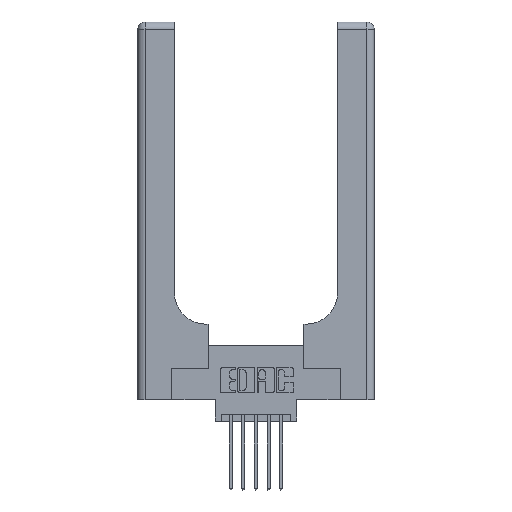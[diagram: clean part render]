
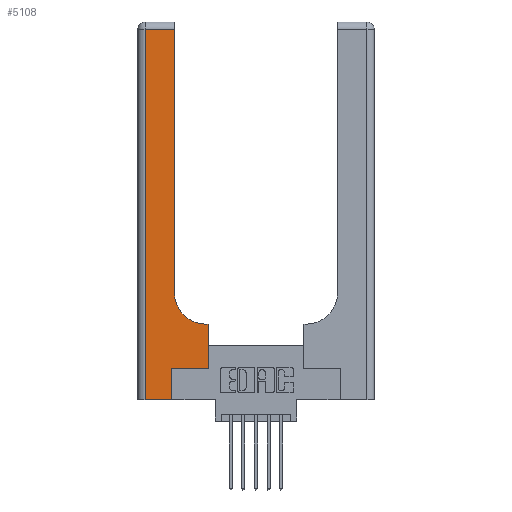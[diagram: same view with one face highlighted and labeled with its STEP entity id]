
A CAD part, top view. The second image highlights one B-rep face of the part: STEP entity #5108.
In plain terms, the highlighted planar face has unit normal (0, 0, 1).
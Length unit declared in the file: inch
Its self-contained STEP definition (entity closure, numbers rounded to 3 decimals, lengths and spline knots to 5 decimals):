
#667 = EDGE_CURVE ( 'NONE', #873, #13312, #13316, .T. ) ;
#873 = VERTEX_POINT ( 'NONE', #10193 ) ;
#890 = VECTOR ( 'NONE', #1889, 39.37008 ) ;
#1004 = VECTOR ( 'NONE', #8299, 39.37008 ) ;
#1135 = DIRECTION ( 'NONE',  ( -1., 0., 0. ) ) ;
#1492 = VECTOR ( 'NONE', #5512, 39.37008 ) ;
#1509 = ORIENTED_EDGE ( 'NONE', *, *, #4184, .T. ) ;
#1645 = CARTESIAN_POINT ( 'NONE',  ( 0.5585, 0.25, 0.37 ) ) ;
#1889 = DIRECTION ( 'NONE',  ( 0., 1., 0. ) ) ;
#2046 = LINE ( 'NONE', #1645, #9063 ) ;
#2167 = EDGE_CURVE ( 'NONE', #13312, #11450, #8857, .T. ) ;
#2388 = CARTESIAN_POINT ( 'NONE',  ( 0.269, 0., 0.37 ) ) ;
#2392 = LINE ( 'NONE', #10535, #1004 ) ;
#2447 = AXIS2_PLACEMENT_3D ( 'NONE', #11686, #13950, #7360 ) ;
#2586 = VERTEX_POINT ( 'NONE', #9330 ) ;
#2750 = DIRECTION ( 'NONE',  ( 0., 1., 0. ) ) ;
#2812 = EDGE_CURVE ( 'NONE', #9667, #2876, #4228, .T. ) ;
#2876 = VERTEX_POINT ( 'NONE', #13076 ) ;
#3674 = CARTESIAN_POINT ( 'NONE',  ( 0.5415, 0.6, 0.37 ) ) ;
#3947 = CARTESIAN_POINT ( 'NONE',  ( 0.2915, 3., 0.37 ) ) ;
#3962 = PLANE ( 'NONE',  #2447 ) ;
#3976 = LINE ( 'NONE', #3947, #890 ) ;
#4128 = CARTESIAN_POINT ( 'NONE',  ( 0.269, 0., 0.37 ) ) ;
#4184 = EDGE_CURVE ( 'NONE', #2876, #4301, #12927, .T. ) ;
#4220 = DIRECTION ( 'NONE',  ( 0., 0., -1. ) ) ;
#4228 = LINE ( 'NONE', #2388, #9704 ) ;
#4301 = VERTEX_POINT ( 'NONE', #10917 ) ;
#4571 = DIRECTION ( 'NONE',  ( -1., 0., 0. ) ) ;
#4712 = EDGE_CURVE ( 'NONE', #8483, #7875, #13614, .T. ) ;
#4749 = ORIENTED_EDGE ( 'NONE', *, *, #10694, .T. ) ;
#5108 = ADVANCED_FACE ( 'NONE', ( #12391 ), #3962, .F. ) ;
#5141 = CARTESIAN_POINT ( 'NONE',  ( 0.06, 3., 0.37 ) ) ;
#5220 = EDGE_CURVE ( 'NONE', #7875, #2586, #10843, .T. ) ;
#5391 = AXIS2_PLACEMENT_3D ( 'NONE', #10932, #4220, #12980 ) ;
#5512 = DIRECTION ( 'NONE',  ( 0., -1., 0. ) ) ;
#5524 = CARTESIAN_POINT ( 'NONE',  ( 0.2915, 0.6, 0.37 ) ) ;
#5591 = ORIENTED_EDGE ( 'NONE', *, *, #667, .T. ) ;
#5715 = EDGE_LOOP ( 'NONE', ( #13948, #5591, #6197, #4749, #6729, #1509, #12548, #10496, #7240 ) ) ;
#5994 = CARTESIAN_POINT ( 'NONE',  ( 0.269, 0.25, 0.37 ) ) ;
#6197 = ORIENTED_EDGE ( 'NONE', *, *, #2167, .T. ) ;
#6718 = EDGE_CURVE ( 'NONE', #4301, #8483, #2046, .T. ) ;
#6729 = ORIENTED_EDGE ( 'NONE', *, *, #2812, .T. ) ;
#6895 = DIRECTION ( 'NONE',  ( 0., 1., 0. ) ) ;
#7240 = ORIENTED_EDGE ( 'NONE', *, *, #5220, .T. ) ;
#7360 = DIRECTION ( 'NONE',  ( -1., 0., 0. ) ) ;
#7875 = VERTEX_POINT ( 'NONE', #3674 ) ;
#8147 = CARTESIAN_POINT ( 'NONE',  ( 0.06, 2.94, 0.37 ) ) ;
#8164 = DIRECTION ( 'NONE',  ( 1., 0., 0. ) ) ;
#8299 = DIRECTION ( 'NONE',  ( 1., 0., 0. ) ) ;
#8483 = VERTEX_POINT ( 'NONE', #11341 ) ;
#8857 = LINE ( 'NONE', #5141, #1492 ) ;
#9063 = VECTOR ( 'NONE', #2750, 39.37008 ) ;
#9077 = EDGE_CURVE ( 'NONE', #2586, #873, #3976, .T. ) ;
#9330 = CARTESIAN_POINT ( 'NONE',  ( 0.2915, 0.85, 0.37 ) ) ;
#9659 = VECTOR ( 'NONE', #8164, 39.37008 ) ;
#9667 = VERTEX_POINT ( 'NONE', #4128 ) ;
#9704 = VECTOR ( 'NONE', #6895, 39.37008 ) ;
#10193 = CARTESIAN_POINT ( 'NONE',  ( 0.2915, 2.94, 0.37 ) ) ;
#10496 = ORIENTED_EDGE ( 'NONE', *, *, #4712, .T. ) ;
#10535 = CARTESIAN_POINT ( 'NONE',  ( 0., 0., 0.37 ) ) ;
#10694 = EDGE_CURVE ( 'NONE', #11450, #9667, #2392, .T. ) ;
#10843 = CIRCLE ( 'NONE', #5391, 0.25 ) ;
#10911 = VECTOR ( 'NONE', #1135, 39.37008 ) ;
#10917 = CARTESIAN_POINT ( 'NONE',  ( 0.5585, 0.25, 0.37 ) ) ;
#10932 = CARTESIAN_POINT ( 'NONE',  ( 0.5415, 0.85, 0.37 ) ) ;
#10984 = CARTESIAN_POINT ( 'NONE',  ( 0., 2.94, 0.37 ) ) ;
#11341 = CARTESIAN_POINT ( 'NONE',  ( 0.5585, 0.6, 0.37 ) ) ;
#11450 = VERTEX_POINT ( 'NONE', #12997 ) ;
#11686 = CARTESIAN_POINT ( 'NONE',  ( 0., 3., 0.37 ) ) ;
#12391 = FACE_OUTER_BOUND ( 'NONE', #5715, .T. ) ;
#12548 = ORIENTED_EDGE ( 'NONE', *, *, #6718, .T. ) ;
#12927 = LINE ( 'NONE', #5994, #9659 ) ;
#12980 = DIRECTION ( 'NONE',  ( 1., 0., 0. ) ) ;
#12997 = CARTESIAN_POINT ( 'NONE',  ( 0.06, 0., 0.37 ) ) ;
#13076 = CARTESIAN_POINT ( 'NONE',  ( 0.269, 0.25, 0.37 ) ) ;
#13312 = VERTEX_POINT ( 'NONE', #8147 ) ;
#13316 = LINE ( 'NONE', #10984, #10911 ) ;
#13614 = LINE ( 'NONE', #5524, #13957 ) ;
#13948 = ORIENTED_EDGE ( 'NONE', *, *, #9077, .T. ) ;
#13950 = DIRECTION ( 'NONE',  ( 0., 0., -1. ) ) ;
#13957 = VECTOR ( 'NONE', #4571, 39.37008 ) ;
